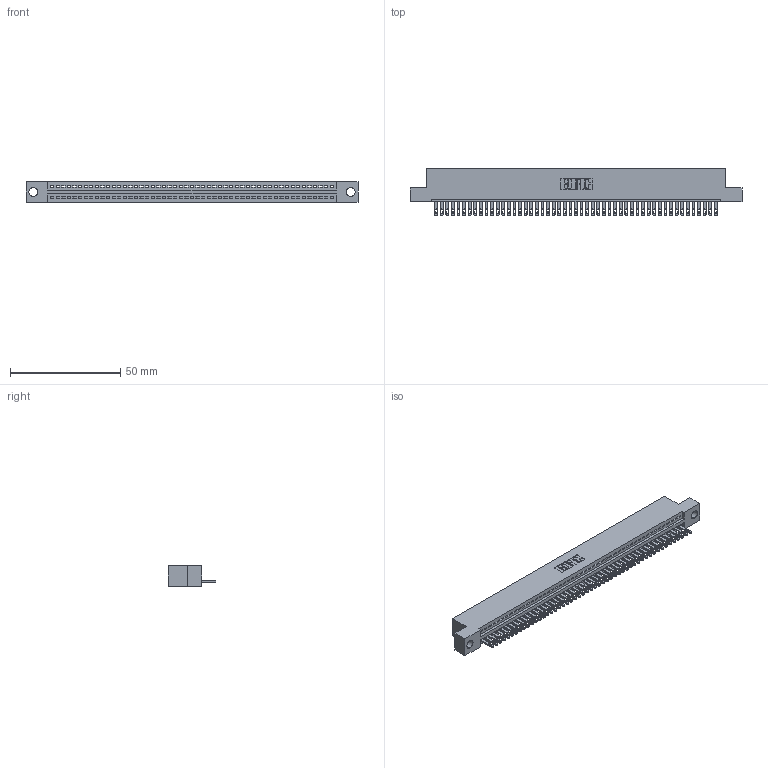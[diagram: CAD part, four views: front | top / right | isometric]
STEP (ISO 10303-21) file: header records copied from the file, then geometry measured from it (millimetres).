
FILE_DESCRIPTION (( 'STEP AP203' ), '1' );
FILE_NAME ('345-051-500-104.STEP', '2019-10-09T13:50:48', ( '' ), ( '' ), 'SwSTEP 2.0', 'SolidWorks 2016', '' );
FILE_SCHEMA (( 'CONFIG_CONTROL_DESIGN' ));
Length unit declared in the file: inch
Products named in the file (3): 345 Part_Flush Mounting Lugs - 0.156 Dia-TH; 345-051-500-104; 345-292-001_345-293-100
Assembly tree (52 placements, depth 2):
  345-051-500-104
    345 Part_Flush Mounting Lugs - 0.156 Dia-TH
    345-292-001_345-293-100  x51
Bounding box: 150.75 x 21.51 x 9.4 mm (x, y, z)
Volume: 14335.7 mm3; surface area: 19096.5 mm2
Topology: 52 solids, 52 shells, 2880 faces, 8909 edges, 5938 vertices
Faces by surface type: plane 1814, cylinder 1066
Entity records: 37105 total; most frequent: CARTESIAN_POINT 6433, ORIENTED_EDGE 6418, DIRECTION 5607, EDGE_CURVE 3209, VECTOR 2869, LINE 2869, VERTEX_POINT 2138, AXIS2_PLACEMENT_3D 1369
